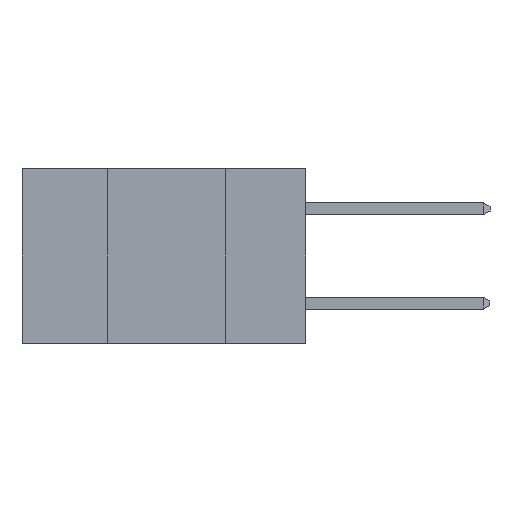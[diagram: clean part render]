
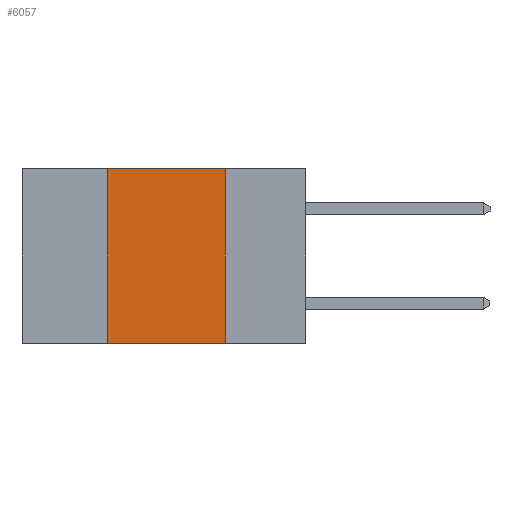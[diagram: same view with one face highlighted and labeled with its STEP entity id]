
A CAD part, left-side view. The second image highlights one B-rep face of the part: STEP entity #6057.
In plain terms, the highlighted planar face has unit normal (-1, 0, 0).
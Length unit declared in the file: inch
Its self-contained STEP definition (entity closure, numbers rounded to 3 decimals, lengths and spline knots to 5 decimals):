
#55 = EDGE_CURVE ( 'NONE', #2547, #976, #7916, .T. ) ;
#159 = VECTOR ( 'NONE', #3702, 39.37008 ) ;
#220 = CARTESIAN_POINT ( 'NONE',  ( 0., 0.6, 0. ) ) ;
#458 = ORIENTED_EDGE ( 'NONE', *, *, #20207, .F. ) ;
#976 = VERTEX_POINT ( 'NONE', #16997 ) ;
#1318 = LINE ( 'NONE', #21940, #159 ) ;
#2199 = DIRECTION ( 'NONE',  ( 0., -1., 0. ) ) ;
#2547 = VERTEX_POINT ( 'NONE', #2749 ) ;
#2749 = CARTESIAN_POINT ( 'NONE',  ( 0., 0.42, -0.37 ) ) ;
#3061 = VECTOR ( 'NONE', #7381, 39.37008 ) ;
#3580 = EDGE_CURVE ( 'NONE', #12157, #21670, #23470, .T. ) ;
#3702 = DIRECTION ( 'NONE',  ( 0., 0., 1. ) ) ;
#5205 = VECTOR ( 'NONE', #2199, 39.37008 ) ;
#5509 = CARTESIAN_POINT ( 'NONE',  ( 0., 0.42, 0. ) ) ;
#5571 = CARTESIAN_POINT ( 'NONE',  ( 0., 0.17, 0. ) ) ;
#6057 = ADVANCED_FACE ( 'NONE', ( #19759 ), #14847, .F. ) ;
#7381 = DIRECTION ( 'NONE',  ( 0., 0., -1. ) ) ;
#7916 = LINE ( 'NONE', #20689, #17193 ) ;
#10877 = ORIENTED_EDGE ( 'NONE', *, *, #3580, .F. ) ;
#12046 = ORIENTED_EDGE ( 'NONE', *, *, #21401, .F. ) ;
#12157 = VERTEX_POINT ( 'NONE', #5509 ) ;
#14847 = PLANE ( 'NONE',  #16166 ) ;
#15855 = DIRECTION ( 'NONE',  ( 1., 0., 0. ) ) ;
#15932 = CARTESIAN_POINT ( 'NONE',  ( 0., 0.6, 0. ) ) ;
#16166 = AXIS2_PLACEMENT_3D ( 'NONE', #15932, #15855, #22373 ) ;
#16313 = DIRECTION ( 'NONE',  ( 0., -1., 0. ) ) ;
#16997 = CARTESIAN_POINT ( 'NONE',  ( 0., 0.17, -0.37 ) ) ;
#17193 = VECTOR ( 'NONE', #16313, 39.37008 ) ;
#17322 = CARTESIAN_POINT ( 'NONE',  ( 0., 0.17, 0. ) ) ;
#17772 = LINE ( 'NONE', #5571, #3061 ) ;
#19759 = FACE_OUTER_BOUND ( 'NONE', #23640, .T. ) ;
#20207 = EDGE_CURVE ( 'NONE', #21670, #976, #17772, .T. ) ;
#20689 = CARTESIAN_POINT ( 'NONE',  ( 0., 0.6, -0.37 ) ) ;
#21401 = EDGE_CURVE ( 'NONE', #2547, #12157, #1318, .T. ) ;
#21670 = VERTEX_POINT ( 'NONE', #17322 ) ;
#21940 = CARTESIAN_POINT ( 'NONE',  ( 0., 0.42, 0. ) ) ;
#22242 = ORIENTED_EDGE ( 'NONE', *, *, #55, .T. ) ;
#22373 = DIRECTION ( 'NONE',  ( 0., 0., -1. ) ) ;
#23470 = LINE ( 'NONE', #220, #5205 ) ;
#23640 = EDGE_LOOP ( 'NONE', ( #458, #10877, #12046, #22242 ) ) ;
